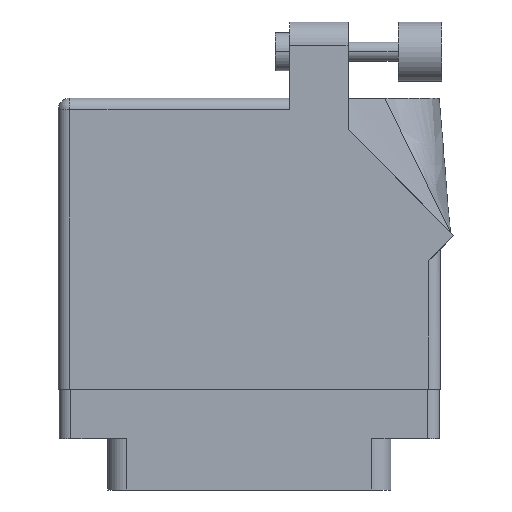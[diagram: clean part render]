
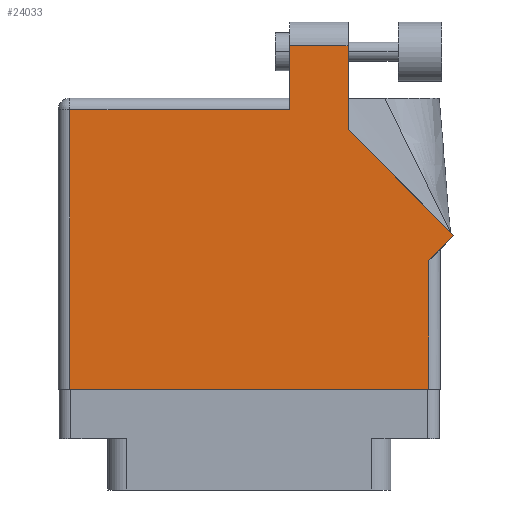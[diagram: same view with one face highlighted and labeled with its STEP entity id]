
A CAD part, front view. The second image highlights one B-rep face of the part: STEP entity #24033.
In plain terms, the highlighted face is planar.
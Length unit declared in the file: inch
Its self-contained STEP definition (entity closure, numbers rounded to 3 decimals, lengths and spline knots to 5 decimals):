
#64 = DIRECTION ( 'NONE',  ( -1., 0., 0. ) ) ;
#217 = VECTOR ( 'NONE', #18699, 39.37008 ) ;
#682 = VERTEX_POINT ( 'NONE', #27439 ) ;
#783 = DIRECTION ( 'NONE',  ( 1., 0., 0. ) ) ;
#941 = VECTOR ( 'NONE', #64, 39.37008 ) ;
#1751 = ORIENTED_EDGE ( 'NONE', *, *, #18259, .T. ) ;
#2028 = VECTOR ( 'NONE', #783, 39.37008 ) ;
#2427 = VECTOR ( 'NONE', #7559, 39.37008 ) ;
#2991 = LINE ( 'NONE', #26696, #17826 ) ;
#3070 = ORIENTED_EDGE ( 'NONE', *, *, #33854, .T. ) ;
#3085 = CARTESIAN_POINT ( 'NONE',  ( 2.01, 0.737, 0. ) ) ;
#3124 = EDGE_CURVE ( 'NONE', #3760, #23817, #27797, .T. ) ;
#3134 = CARTESIAN_POINT ( 'NONE',  ( 1.217, 1.53, 0. ) ) ;
#3760 = VERTEX_POINT ( 'NONE', #15373 ) ;
#4226 = EDGE_CURVE ( 'NONE', #10227, #682, #29258, .T. ) ;
#5225 = CARTESIAN_POINT ( 'NONE',  ( 2.08071, 0.80771, 0. ) ) ;
#5372 = CARTESIAN_POINT ( 'NONE',  ( 1.217, 1.805, 0. ) ) ;
#6854 = LINE ( 'NONE', #17624, #10253 ) ;
#7273 = ORIENTED_EDGE ( 'NONE', *, *, #4226, .T. ) ;
#7441 = ORIENTED_EDGE ( 'NONE', *, *, #32784, .T. ) ;
#7559 = DIRECTION ( 'NONE',  ( 0., 1., 0. ) ) ;
#7619 = VERTEX_POINT ( 'NONE', #26564 ) ;
#8254 = ORIENTED_EDGE ( 'NONE', *, *, #14842, .T. ) ;
#8437 = LINE ( 'NONE', #3134, #217 ) ;
#8904 = CARTESIAN_POINT ( 'NONE',  ( 1.948, 0.737, 0. ) ) ;
#9427 = LINE ( 'NONE', #3085, #11681 ) ;
#9552 = FACE_OUTER_BOUND ( 'NONE', #13950, .T. ) ;
#9697 = LINE ( 'NONE', #31254, #2427 ) ;
#10227 = VERTEX_POINT ( 'NONE', #19341 ) ;
#10253 = VECTOR ( 'NONE', #11622, 39.37008 ) ;
#10528 = AXIS2_PLACEMENT_3D ( 'NONE', #30940, #33939, #23508 ) ;
#11622 = DIRECTION ( 'NONE',  ( 0., -1., 0. ) ) ;
#11681 = VECTOR ( 'NONE', #30979, 39.37008 ) ;
#12394 = VERTEX_POINT ( 'NONE', #18200 ) ;
#12422 = LINE ( 'NONE', #34337, #15516 ) ;
#13950 = EDGE_LOOP ( 'NONE', ( #7441, #7273, #3070, #1751, #27341, #28624, #16494, #17444, #8254 ) ) ;
#14842 = EDGE_CURVE ( 'NONE', #27594, #7619, #12422, .T. ) ;
#15032 = PLANE ( 'NONE',  #10528 ) ;
#15373 = CARTESIAN_POINT ( 'NONE',  ( 1.948, 0., 0. ) ) ;
#15516 = VECTOR ( 'NONE', #23377, 39.37008 ) ;
#16494 = ORIENTED_EDGE ( 'NONE', *, *, #3124, .T. ) ;
#17043 = CARTESIAN_POINT ( 'NONE',  ( 0., 0., 0. ) ) ;
#17444 = ORIENTED_EDGE ( 'NONE', *, *, #19220, .T. ) ;
#17624 = CARTESIAN_POINT ( 'NONE',  ( 0.062, 0., 0. ) ) ;
#17826 = VECTOR ( 'NONE', #24385, 39.37008 ) ;
#18200 = CARTESIAN_POINT ( 'NONE',  ( 1.217, 1.468, 0. ) ) ;
#18259 = EDGE_CURVE ( 'NONE', #12394, #29299, #2991, .T. ) ;
#18699 = DIRECTION ( 'NONE',  ( 0., -1., 0. ) ) ;
#19192 = VERTEX_POINT ( 'NONE', #27660 ) ;
#19220 = EDGE_CURVE ( 'NONE', #23817, #27594, #9427, .T. ) ;
#19341 = CARTESIAN_POINT ( 'NONE',  ( 1.524, 1.805, 0. ) ) ;
#23127 = EDGE_CURVE ( 'NONE', #19192, #3760, #30856, .T. ) ;
#23377 = DIRECTION ( 'NONE',  ( -0.707, 0.707, 0. ) ) ;
#23508 = DIRECTION ( 'NONE',  ( -1., 0., 0. ) ) ;
#23817 = VERTEX_POINT ( 'NONE', #32696 ) ;
#24033 = ADVANCED_FACE ( 'NONE', ( #9552 ), #15032, .F. ) ;
#24105 = VECTOR ( 'NONE', #30459, 39.37008 ) ;
#24385 = DIRECTION ( 'NONE',  ( -1., 0., 0. ) ) ;
#26564 = CARTESIAN_POINT ( 'NONE',  ( 1.524, 1.36442, 0. ) ) ;
#26696 = CARTESIAN_POINT ( 'NONE',  ( 0., 1.468, 0. ) ) ;
#27341 = ORIENTED_EDGE ( 'NONE', *, *, #27365, .T. ) ;
#27365 = EDGE_CURVE ( 'NONE', #29299, #19192, #6854, .T. ) ;
#27439 = CARTESIAN_POINT ( 'NONE',  ( 1.217, 1.805, 0. ) ) ;
#27594 = VERTEX_POINT ( 'NONE', #5225 ) ;
#27660 = CARTESIAN_POINT ( 'NONE',  ( 0.062, 0., 0. ) ) ;
#27797 = LINE ( 'NONE', #8904, #24105 ) ;
#28624 = ORIENTED_EDGE ( 'NONE', *, *, #23127, .T. ) ;
#29258 = LINE ( 'NONE', #5372, #941 ) ;
#29299 = VERTEX_POINT ( 'NONE', #33808 ) ;
#30459 = DIRECTION ( 'NONE',  ( 0., 1., 0. ) ) ;
#30856 = LINE ( 'NONE', #17043, #2028 ) ;
#30940 = CARTESIAN_POINT ( 'NONE',  ( 0., 1.53, 0. ) ) ;
#30979 = DIRECTION ( 'NONE',  ( 0.707, 0.707, 0. ) ) ;
#31254 = CARTESIAN_POINT ( 'NONE',  ( 1.524, 1.36442, 0. ) ) ;
#32696 = CARTESIAN_POINT ( 'NONE',  ( 1.948, 0.675, 0. ) ) ;
#32784 = EDGE_CURVE ( 'NONE', #7619, #10227, #9697, .T. ) ;
#33808 = CARTESIAN_POINT ( 'NONE',  ( 0.062, 1.468, 0. ) ) ;
#33854 = EDGE_CURVE ( 'NONE', #682, #12394, #8437, .T. ) ;
#33939 = DIRECTION ( 'NONE',  ( 0., 0., -1. ) ) ;
#34337 = CARTESIAN_POINT ( 'NONE',  ( 2.08071, 0.80771, 0. ) ) ;
